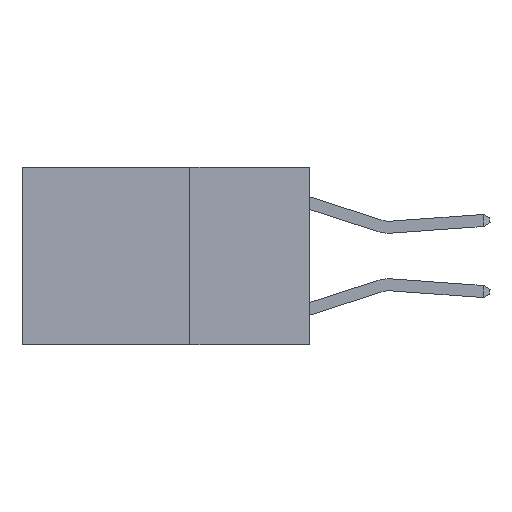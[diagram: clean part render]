
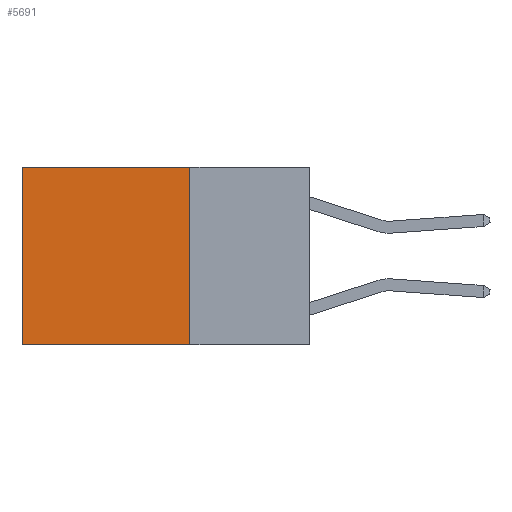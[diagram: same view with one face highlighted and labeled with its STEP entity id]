
A CAD part, left-side view. The second image highlights one B-rep face of the part: STEP entity #5691.
In plain terms, the highlighted planar face has unit normal (-1, 0, 0).
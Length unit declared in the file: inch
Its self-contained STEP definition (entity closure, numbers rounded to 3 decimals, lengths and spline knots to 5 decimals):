
#55 = VECTOR ( 'NONE', #7908, 39.37008 ) ;
#408 = VERTEX_POINT ( 'NONE', #784 ) ;
#464 = DIRECTION ( 'NONE',  ( 0., 1., 0. ) ) ;
#745 = ORIENTED_EDGE ( 'NONE', *, *, #9641, .T. ) ;
#784 = CARTESIAN_POINT ( 'NONE',  ( 0.2625, 0.25, 0. ) ) ;
#1841 = VERTEX_POINT ( 'NONE', #10274 ) ;
#1874 = CARTESIAN_POINT ( 'NONE',  ( 0.2625, 0.25, 0. ) ) ;
#1935 = ORIENTED_EDGE ( 'NONE', *, *, #11955, .T. ) ;
#2419 = FACE_OUTER_BOUND ( 'NONE', #3760, .T. ) ;
#3342 = CARTESIAN_POINT ( 'NONE',  ( 0.2625, 0.25, -0.37 ) ) ;
#3531 = CARTESIAN_POINT ( 'NONE',  ( 0.2625, 0.25, 0. ) ) ;
#3577 = ORIENTED_EDGE ( 'NONE', *, *, #11431, .F. ) ;
#3604 = LINE ( 'NONE', #10615, #11900 ) ;
#3760 = EDGE_LOOP ( 'NONE', ( #1935, #3577, #11101, #745 ) ) ;
#4530 = LINE ( 'NONE', #8040, #8747 ) ;
#4541 = LINE ( 'NONE', #3531, #11077 ) ;
#4784 = DIRECTION ( 'NONE',  ( 0., 0., -1. ) ) ;
#5691 = ADVANCED_FACE ( 'NONE', ( #2419 ), #9374, .F. ) ;
#6553 = VERTEX_POINT ( 'NONE', #12606 ) ;
#7284 = DIRECTION ( 'NONE',  ( 0., 0., -1. ) ) ;
#7417 = CARTESIAN_POINT ( 'NONE',  ( 0.2625, 0.25, 0. ) ) ;
#7543 = DIRECTION ( 'NONE',  ( 0., 1., 0. ) ) ;
#7724 = AXIS2_PLACEMENT_3D ( 'NONE', #7417, #8514, #7284 ) ;
#7908 = DIRECTION ( 'NONE',  ( 0., 0., -1. ) ) ;
#8040 = CARTESIAN_POINT ( 'NONE',  ( 0.2625, 0.6, 0. ) ) ;
#8514 = DIRECTION ( 'NONE',  ( 1., 0., 0. ) ) ;
#8747 = VECTOR ( 'NONE', #4784, 39.37008 ) ;
#8938 = LINE ( 'NONE', #1874, #55 ) ;
#9268 = VERTEX_POINT ( 'NONE', #3342 ) ;
#9374 = PLANE ( 'NONE',  #7724 ) ;
#9641 = EDGE_CURVE ( 'NONE', #408, #1841, #4541, .T. ) ;
#10274 = CARTESIAN_POINT ( 'NONE',  ( 0.2625, 0.6, 0. ) ) ;
#10615 = CARTESIAN_POINT ( 'NONE',  ( 0.2625, 0.25, -0.37 ) ) ;
#11077 = VECTOR ( 'NONE', #464, 39.37008 ) ;
#11101 = ORIENTED_EDGE ( 'NONE', *, *, #12067, .F. ) ;
#11431 = EDGE_CURVE ( 'NONE', #9268, #6553, #3604, .T. ) ;
#11900 = VECTOR ( 'NONE', #7543, 39.37008 ) ;
#11955 = EDGE_CURVE ( 'NONE', #1841, #6553, #4530, .T. ) ;
#12067 = EDGE_CURVE ( 'NONE', #408, #9268, #8938, .T. ) ;
#12606 = CARTESIAN_POINT ( 'NONE',  ( 0.2625, 0.6, -0.37 ) ) ;
